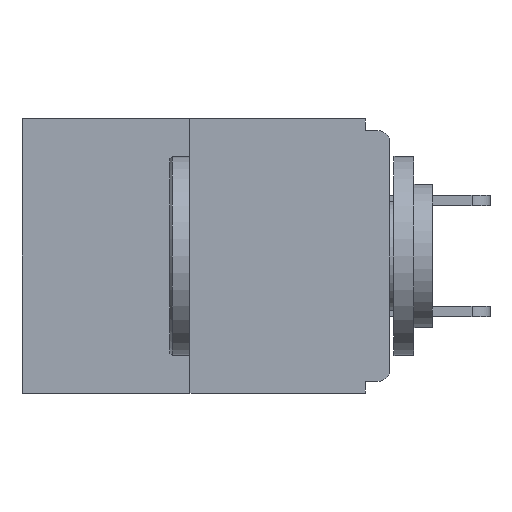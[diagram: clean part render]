
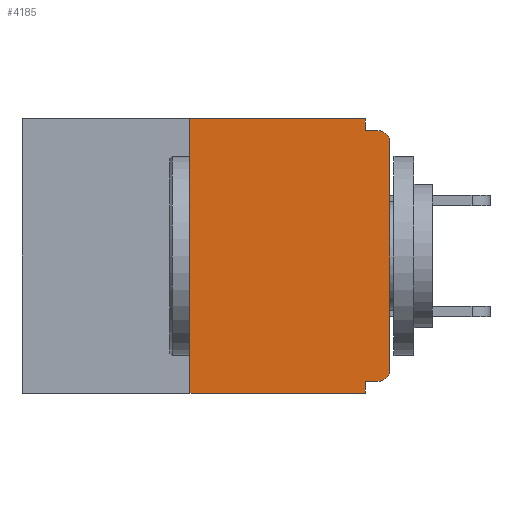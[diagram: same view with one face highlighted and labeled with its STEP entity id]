
A CAD part, left-side view. The second image highlights one B-rep face of the part: STEP entity #4185.
In plain terms, the highlighted planar face has unit normal (-1, 0, 0).
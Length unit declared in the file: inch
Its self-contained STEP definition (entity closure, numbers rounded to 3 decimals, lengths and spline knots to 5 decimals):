
#88 = AXIS2_PLACEMENT_3D ( 'NONE', #12547, #4351, #2836 ) ;
#164 = ORIENTED_EDGE ( 'NONE', *, *, #2329, .F. ) ;
#267 = VERTEX_POINT ( 'NONE', #319 ) ;
#281 = VERTEX_POINT ( 'NONE', #16610 ) ;
#319 = CARTESIAN_POINT ( 'NONE',  ( 0., 0., -0.313 ) ) ;
#432 = EDGE_CURVE ( 'NONE', #10386, #9559, #14361, .T. ) ;
#437 = DIRECTION ( 'NONE',  ( 0., 0., 1. ) ) ;
#1516 = ORIENTED_EDGE ( 'NONE', *, *, #9022, .F. ) ;
#1553 = VECTOR ( 'NONE', #15226, 39.37008 ) ;
#1577 = ORIENTED_EDGE ( 'NONE', *, *, #11715, .F. ) ;
#1821 = VECTOR ( 'NONE', #12673, 39.37008 ) ;
#2103 = DIRECTION ( 'NONE',  ( 0., 0., 1. ) ) ;
#2251 = ORIENTED_EDGE ( 'NONE', *, *, #6237, .T. ) ;
#2329 = EDGE_CURVE ( 'NONE', #11182, #281, #11125, .T. ) ;
#2836 = DIRECTION ( 'NONE',  ( 0., 0., -1. ) ) ;
#2902 = DIRECTION ( 'NONE',  ( 0., 0., -1. ) ) ;
#2933 = CARTESIAN_POINT ( 'NONE',  ( 0., 0.015, -0.328 ) ) ;
#3007 = EDGE_CURVE ( 'NONE', #3247, #267, #3840, .T. ) ;
#3235 = CARTESIAN_POINT ( 'NONE',  ( 0., 0., 0. ) ) ;
#3247 = VERTEX_POINT ( 'NONE', #2933 ) ;
#3633 = CARTESIAN_POINT ( 'NONE',  ( 0., 0.015, -0.313 ) ) ;
#3839 = VECTOR ( 'NONE', #10387, 39.37008 ) ;
#3840 = CIRCLE ( 'NONE', #16465, 0.015 ) ;
#4070 = VERTEX_POINT ( 'NONE', #4685 ) ;
#4113 = PLANE ( 'NONE',  #88 ) ;
#4185 = ADVANCED_FACE ( 'NONE', ( #14273 ), #4113, .F. ) ;
#4351 = DIRECTION ( 'NONE',  ( 1., 0., 0. ) ) ;
#4593 = CIRCLE ( 'NONE', #10498, 0.015 ) ;
#4684 = LINE ( 'NONE', #3235, #8554 ) ;
#4685 = CARTESIAN_POINT ( 'NONE',  ( 0., 0.015, -0.015 ) ) ;
#4983 = CARTESIAN_POINT ( 'NONE',  ( 0., 0., -0.03 ) ) ;
#5130 = DIRECTION ( 'NONE',  ( 0., -1., 0. ) ) ;
#5222 = VECTOR ( 'NONE', #11122, 39.37008 ) ;
#5469 = CARTESIAN_POINT ( 'NONE',  ( 0., 0.25, -0.343 ) ) ;
#5506 = LINE ( 'NONE', #15979, #12985 ) ;
#6158 = EDGE_CURVE ( 'NONE', #3247, #11182, #8020, .T. ) ;
#6237 = EDGE_CURVE ( 'NONE', #16063, #4070, #4593, .T. ) ;
#6444 = CARTESIAN_POINT ( 'NONE',  ( 0., 0.031, -0.343 ) ) ;
#7541 = ORIENTED_EDGE ( 'NONE', *, *, #14726, .T. ) ;
#7812 = LINE ( 'NONE', #8966, #13147 ) ;
#8020 = LINE ( 'NONE', #16501, #5222 ) ;
#8554 = VECTOR ( 'NONE', #437, 39.37008 ) ;
#8966 = CARTESIAN_POINT ( 'NONE',  ( 0., 0.25, 0. ) ) ;
#9022 = EDGE_CURVE ( 'NONE', #12365, #10386, #5506, .T. ) ;
#9442 = LINE ( 'NONE', #11175, #1553 ) ;
#9559 = VERTEX_POINT ( 'NONE', #10470 ) ;
#9992 = ORIENTED_EDGE ( 'NONE', *, *, #6158, .F. ) ;
#10386 = VERTEX_POINT ( 'NONE', #13883 ) ;
#10387 = DIRECTION ( 'NONE',  ( 0., 0., -1. ) ) ;
#10470 = CARTESIAN_POINT ( 'NONE',  ( 0., 0.031, -0.015 ) ) ;
#10479 = ORIENTED_EDGE ( 'NONE', *, *, #3007, .T. ) ;
#10498 = AXIS2_PLACEMENT_3D ( 'NONE', #13673, #13609, #2902 ) ;
#10792 = LINE ( 'NONE', #13389, #17156 ) ;
#10846 = ORIENTED_EDGE ( 'NONE', *, *, #13450, .T. ) ;
#10905 = ORIENTED_EDGE ( 'NONE', *, *, #11209, .F. ) ;
#11122 = DIRECTION ( 'NONE',  ( 0., 1., 0. ) ) ;
#11125 = LINE ( 'NONE', #6444, #3839 ) ;
#11175 = CARTESIAN_POINT ( 'NONE',  ( 0., 0.46, -0.343 ) ) ;
#11182 = VERTEX_POINT ( 'NONE', #12892 ) ;
#11209 = EDGE_CURVE ( 'NONE', #14552, #12365, #7812, .T. ) ;
#11715 = EDGE_CURVE ( 'NONE', #9559, #4070, #10792, .T. ) ;
#12365 = VERTEX_POINT ( 'NONE', #12955 ) ;
#12547 = CARTESIAN_POINT ( 'NONE',  ( 0., 0.46, 0. ) ) ;
#12673 = DIRECTION ( 'NONE',  ( 0., 0., -1. ) ) ;
#12892 = CARTESIAN_POINT ( 'NONE',  ( 0., 0.031, -0.328 ) ) ;
#12955 = CARTESIAN_POINT ( 'NONE',  ( 0., 0.25, 0. ) ) ;
#12985 = VECTOR ( 'NONE', #5130, 39.37008 ) ;
#13020 = ORIENTED_EDGE ( 'NONE', *, *, #432, .F. ) ;
#13147 = VECTOR ( 'NONE', #2103, 39.37008 ) ;
#13389 = CARTESIAN_POINT ( 'NONE',  ( 0., 0., -0.015 ) ) ;
#13450 = EDGE_CURVE ( 'NONE', #14552, #281, #9442, .T. ) ;
#13609 = DIRECTION ( 'NONE',  ( -1., 0., 0. ) ) ;
#13673 = CARTESIAN_POINT ( 'NONE',  ( 0., 0.015, -0.03 ) ) ;
#13789 = CARTESIAN_POINT ( 'NONE',  ( 0., 0.031, 0. ) ) ;
#13883 = CARTESIAN_POINT ( 'NONE',  ( 0., 0.031, 0. ) ) ;
#14273 = FACE_OUTER_BOUND ( 'NONE', #16633, .T. ) ;
#14361 = LINE ( 'NONE', #13789, #1821 ) ;
#14552 = VERTEX_POINT ( 'NONE', #5469 ) ;
#14578 = DIRECTION ( 'NONE',  ( -1., 0., 0. ) ) ;
#14726 = EDGE_CURVE ( 'NONE', #267, #16063, #4684, .T. ) ;
#15226 = DIRECTION ( 'NONE',  ( 0., -1., 0. ) ) ;
#15871 = DIRECTION ( 'NONE',  ( 0., -1., 0. ) ) ;
#15942 = DIRECTION ( 'NONE',  ( 0., 0., -1. ) ) ;
#15979 = CARTESIAN_POINT ( 'NONE',  ( 0., 0.46, 0. ) ) ;
#16063 = VERTEX_POINT ( 'NONE', #4983 ) ;
#16465 = AXIS2_PLACEMENT_3D ( 'NONE', #3633, #14578, #15942 ) ;
#16501 = CARTESIAN_POINT ( 'NONE',  ( 0., 0., -0.328 ) ) ;
#16610 = CARTESIAN_POINT ( 'NONE',  ( 0., 0.031, -0.343 ) ) ;
#16633 = EDGE_LOOP ( 'NONE', ( #1516, #10905, #10846, #164, #9992, #10479, #7541, #2251, #1577, #13020 ) ) ;
#17156 = VECTOR ( 'NONE', #15871, 39.37008 ) ;
